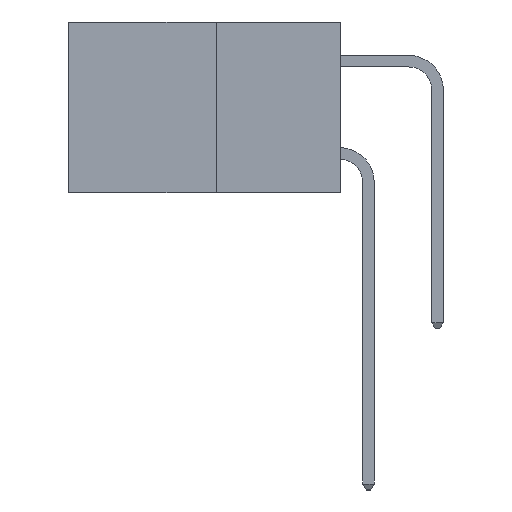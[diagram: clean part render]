
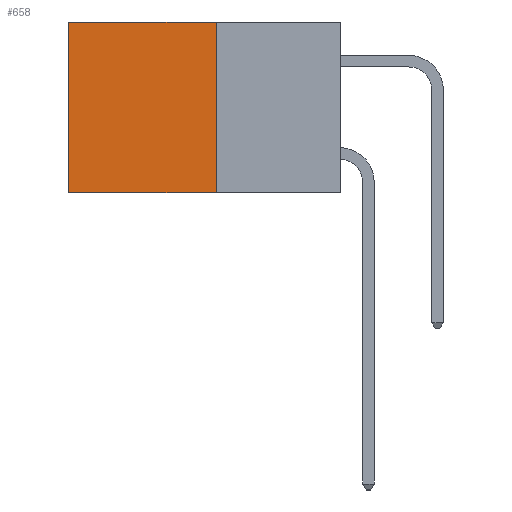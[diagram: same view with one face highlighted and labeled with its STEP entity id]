
A CAD part, left-side view. The second image highlights one B-rep face of the part: STEP entity #658.
In plain terms, the highlighted planar face has unit normal (-1, 0, 0).
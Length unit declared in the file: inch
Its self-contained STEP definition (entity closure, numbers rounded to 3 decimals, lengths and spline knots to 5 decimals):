
#658 = ADVANCED_FACE ( 'NONE', ( #11922 ), #10236, .F. ) ;
#707 = ORIENTED_EDGE ( 'NONE', *, *, #3723, .T. ) ;
#1330 = LINE ( 'NONE', #12413, #12387 ) ;
#1413 = DIRECTION ( 'NONE',  ( 0., 1., 0. ) ) ;
#1872 = EDGE_CURVE ( 'NONE', #11739, #7223, #12200, .T. ) ;
#2081 = DIRECTION ( 'NONE',  ( 0., 0., -1. ) ) ;
#2132 = CARTESIAN_POINT ( 'NONE',  ( 0.277, 0.27, -0.37 ) ) ;
#2134 = CARTESIAN_POINT ( 'NONE',  ( 0.277, 0.27, 0. ) ) ;
#2276 = CARTESIAN_POINT ( 'NONE',  ( 0.277, 0.27, -0.37 ) ) ;
#2297 = AXIS2_PLACEMENT_3D ( 'NONE', #3430, #13362, #10963 ) ;
#2410 = VERTEX_POINT ( 'NONE', #2134 ) ;
#3066 = CARTESIAN_POINT ( 'NONE',  ( 0.277, 0.59, 0. ) ) ;
#3430 = CARTESIAN_POINT ( 'NONE',  ( 0.277, 0.27, -0.37 ) ) ;
#3525 = CARTESIAN_POINT ( 'NONE',  ( 0.277, 0.27, -0.37 ) ) ;
#3723 = EDGE_CURVE ( 'NONE', #2410, #10757, #1330, .T. ) ;
#4520 = EDGE_CURVE ( 'NONE', #10757, #7223, #8590, .T. ) ;
#6870 = VECTOR ( 'NONE', #1413, 39.37008 ) ;
#6981 = CARTESIAN_POINT ( 'NONE',  ( 0.277, 0.59, -0.37 ) ) ;
#7223 = VERTEX_POINT ( 'NONE', #6981 ) ;
#7872 = ORIENTED_EDGE ( 'NONE', *, *, #4520, .T. ) ;
#8495 = ORIENTED_EDGE ( 'NONE', *, *, #1872, .F. ) ;
#8590 = LINE ( 'NONE', #12934, #11268 ) ;
#9463 = VECTOR ( 'NONE', #2081, 39.37008 ) ;
#10103 = LINE ( 'NONE', #2132, #9463 ) ;
#10236 = PLANE ( 'NONE',  #2297 ) ;
#10711 = EDGE_LOOP ( 'NONE', ( #7872, #8495, #11179, #707 ) ) ;
#10757 = VERTEX_POINT ( 'NONE', #3066 ) ;
#10850 = EDGE_CURVE ( 'NONE', #2410, #11739, #10103, .T. ) ;
#10963 = DIRECTION ( 'NONE',  ( 0., 0., -1. ) ) ;
#11179 = ORIENTED_EDGE ( 'NONE', *, *, #10850, .F. ) ;
#11268 = VECTOR ( 'NONE', #12922, 39.37008 ) ;
#11739 = VERTEX_POINT ( 'NONE', #3525 ) ;
#11922 = FACE_OUTER_BOUND ( 'NONE', #10711, .T. ) ;
#12035 = DIRECTION ( 'NONE',  ( 0., 1., 0. ) ) ;
#12200 = LINE ( 'NONE', #2276, #6870 ) ;
#12387 = VECTOR ( 'NONE', #12035, 39.37008 ) ;
#12413 = CARTESIAN_POINT ( 'NONE',  ( 0.277, 0.27, 0. ) ) ;
#12922 = DIRECTION ( 'NONE',  ( 0., 0., -1. ) ) ;
#12934 = CARTESIAN_POINT ( 'NONE',  ( 0.277, 0.59, -0.37 ) ) ;
#13362 = DIRECTION ( 'NONE',  ( 1., 0., 0. ) ) ;
